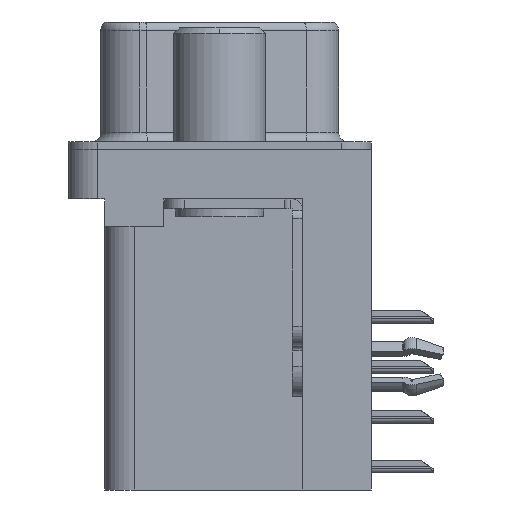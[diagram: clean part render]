
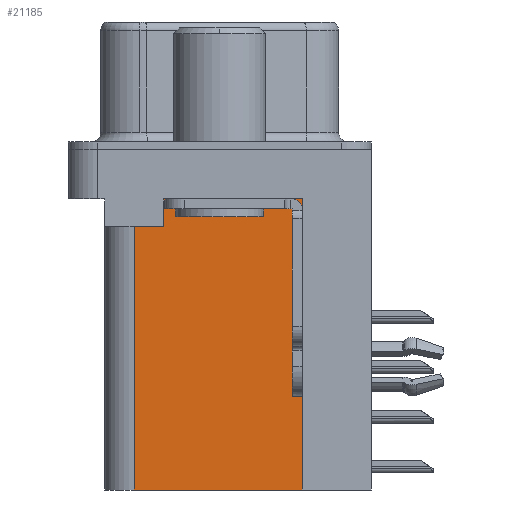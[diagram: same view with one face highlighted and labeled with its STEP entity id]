
A CAD part, left-side view. The second image highlights one B-rep face of the part: STEP entity #21185.
In plain terms, the highlighted planar face has unit normal (-1, 0, 0).
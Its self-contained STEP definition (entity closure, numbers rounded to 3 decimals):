
#979 = CARTESIAN_POINT ( 'NONE',  ( 3.75, 4.35, -17.3 ) ) ;
#1220 = ORIENTED_EDGE ( 'NONE', *, *, #25770, .F. ) ;
#2144 = CARTESIAN_POINT ( 'NONE',  ( 3.75, 4.35, -3.9 ) ) ;
#2667 = VERTEX_POINT ( 'NONE', #5452 ) ;
#2854 = ORIENTED_EDGE ( 'NONE', *, *, #24247, .F. ) ;
#4502 = DIRECTION ( 'NONE',  ( 0., 0., 1. ) ) ;
#4735 = EDGE_CURVE ( 'NONE', #2667, #8137, #25159, .T. ) ;
#5452 = CARTESIAN_POINT ( 'NONE',  ( 3.75, -4.2, -2.5 ) ) ;
#5762 = LINE ( 'NONE', #979, #22417 ) ;
#5783 = VERTEX_POINT ( 'NONE', #17821 ) ;
#6028 = ORIENTED_EDGE ( 'NONE', *, *, #18511, .T. ) ;
#6407 = VECTOR ( 'NONE', #20639, 1000. ) ;
#6768 = DIRECTION ( 'NONE',  ( 0., 0., -1. ) ) ;
#6857 = CARTESIAN_POINT ( 'NONE',  ( 3.75, 2.85, -3.9 ) ) ;
#6910 = EDGE_CURVE ( 'NONE', #8137, #17341, #20758, .T. ) ;
#7210 = EDGE_CURVE ( 'NONE', #17341, #27024, #11331, .T. ) ;
#7570 = DIRECTION ( 'NONE',  ( 0., 1., 0. ) ) ;
#8137 = VERTEX_POINT ( 'NONE', #35611 ) ;
#10496 = CARTESIAN_POINT ( 'NONE',  ( 3.75, -4.2, -17.3 ) ) ;
#11331 = LINE ( 'NONE', #30530, #21270 ) ;
#15486 = VERTEX_POINT ( 'NONE', #10496 ) ;
#15649 = ORIENTED_EDGE ( 'NONE', *, *, #6910, .T. ) ;
#17029 = CARTESIAN_POINT ( 'NONE',  ( 3.75, -4.2, -17.3 ) ) ;
#17341 = VERTEX_POINT ( 'NONE', #34858 ) ;
#17750 = AXIS2_PLACEMENT_3D ( 'NONE', #37570, #27496, #7570 ) ;
#17807 = ORIENTED_EDGE ( 'NONE', *, *, #7210, .T. ) ;
#17821 = CARTESIAN_POINT ( 'NONE',  ( 3.75, 4.35, -17.3 ) ) ;
#18432 = CARTESIAN_POINT ( 'NONE',  ( 3.75, -4.2, -2.5 ) ) ;
#18511 = EDGE_CURVE ( 'NONE', #15486, #2667, #36339, .T. ) ;
#18970 = ORIENTED_EDGE ( 'NONE', *, *, #4735, .T. ) ;
#19344 = CARTESIAN_POINT ( 'NONE',  ( 3.75, -4.2, -17.3 ) ) ;
#20639 = DIRECTION ( 'NONE',  ( 0., 1., 0. ) ) ;
#20758 = LINE ( 'NONE', #6857, #37586 ) ;
#21185 = ADVANCED_FACE ( 'NONE', ( #23492 ), #24201, .F. ) ;
#21270 = VECTOR ( 'NONE', #40644, 1000. ) ;
#22417 = VECTOR ( 'NONE', #4502, 1000. ) ;
#23492 = FACE_OUTER_BOUND ( 'NONE', #31375, .T. ) ;
#24201 = PLANE ( 'NONE',  #17750 ) ;
#24247 = EDGE_CURVE ( 'NONE', #5783, #27024, #5762, .T. ) ;
#25159 = LINE ( 'NONE', #18432, #6407 ) ;
#25770 = EDGE_CURVE ( 'NONE', #15486, #5783, #30683, .T. ) ;
#27024 = VERTEX_POINT ( 'NONE', #2144 ) ;
#27496 = DIRECTION ( 'NONE',  ( 1., 0., 0. ) ) ;
#30530 = CARTESIAN_POINT ( 'NONE',  ( 3.75, 0., -3.9 ) ) ;
#30683 = LINE ( 'NONE', #19344, #40752 ) ;
#31375 = EDGE_LOOP ( 'NONE', ( #18970, #15649, #17807, #2854, #1220, #6028 ) ) ;
#34858 = CARTESIAN_POINT ( 'NONE',  ( 3.75, 2.85, -3.9 ) ) ;
#35266 = VECTOR ( 'NONE', #37169, 1000. ) ;
#35611 = CARTESIAN_POINT ( 'NONE',  ( 3.75, 2.85, -2.5 ) ) ;
#36339 = LINE ( 'NONE', #17029, #35266 ) ;
#37169 = DIRECTION ( 'NONE',  ( 0., 0., 1. ) ) ;
#37570 = CARTESIAN_POINT ( 'NONE',  ( 3.75, -4.2, -17.3 ) ) ;
#37586 = VECTOR ( 'NONE', #6768, 1000. ) ;
#40644 = DIRECTION ( 'NONE',  ( 0., 1., 0. ) ) ;
#40752 = VECTOR ( 'NONE', #42870, 1000. ) ;
#42870 = DIRECTION ( 'NONE',  ( 0., 1., 0. ) ) ;
